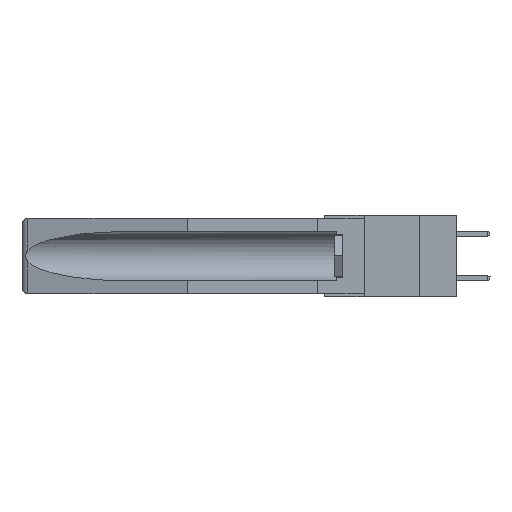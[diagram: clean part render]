
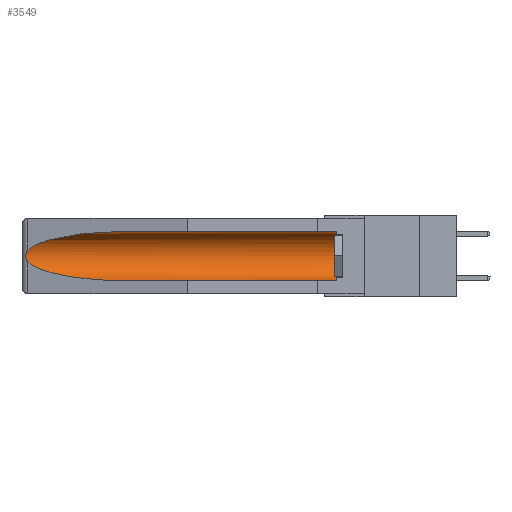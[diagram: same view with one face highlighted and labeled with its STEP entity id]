
A CAD part, left-side view. The second image highlights one B-rep face of the part: STEP entity #3549.
In plain terms, the highlighted cylindrical face has radius 2.857 mm (diameter 5.715 mm), a partial arc.
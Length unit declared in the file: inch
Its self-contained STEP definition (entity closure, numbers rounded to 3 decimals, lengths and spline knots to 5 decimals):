
#280 = CARTESIAN_POINT ( 'NONE',  ( 0.26537, 1.52718, -0.19328 ) ) ;
#306 = DIRECTION ( 'NONE',  ( 0., 1., 0. ) ) ;
#454 = VERTEX_POINT ( 'NONE', #927 ) ;
#563 = CARTESIAN_POINT ( 'NONE',  ( 0.26537, 1.52718, -0.14972 ) ) ;
#865 = DIRECTION ( 'NONE',  ( 0., 1., 0. ) ) ;
#877 = EDGE_LOOP ( 'NONE', ( #3183, #9556, #5149, #1847, #10025, #9889 ) ) ;
#927 = CARTESIAN_POINT ( 'NONE',  ( 0.155, 1.07973, -0.059 ) ) ;
#1046 = CARTESIAN_POINT ( 'NONE',  ( 0.2675, 1.53308, -0.16763 ) ) ;
#1102 = CARTESIAN_POINT ( 'NONE',  ( 0.155, -0.30754, -0.1715 ) ) ;
#1105 = VERTEX_POINT ( 'NONE', #1266 ) ;
#1266 = CARTESIAN_POINT ( 'NONE',  ( 0.155, 0.126, -0.284 ) ) ;
#1847 = ORIENTED_EDGE ( 'NONE', *, *, #3578, .F. ) ;
#2522 = CARTESIAN_POINT ( 'NONE',  ( 0.26597, 1.5296, -0.19026 ) ) ;
#3038 = CARTESIAN_POINT ( 'NONE',  ( 0.155, 0.126, -0.059 ) ) ;
#3183 = ORIENTED_EDGE ( 'NONE', *, *, #11497, .T. ) ;
#3514 = VECTOR ( 'NONE', #306, 39.37008 ) ;
#3549 = ADVANCED_FACE ( 'NONE', ( #17587 ), #16458, .F. ) ;
#3558 = EDGE_CURVE ( 'NONE', #17752, #16629, #10511, .T. ) ;
#3578 = EDGE_CURVE ( 'NONE', #1105, #8417, #11585, .T. ) ;
#3604 = CARTESIAN_POINT ( 'NONE',  ( 0.21114, 1.30732, -0.059 ) ) ;
#3857 = CARTESIAN_POINT ( 'NONE',  ( 0.2675, 1.53308, -0.17534 ) ) ;
#5149 = ORIENTED_EDGE ( 'NONE', *, *, #5478, .T. ) ;
#5207 = CARTESIAN_POINT ( 'NONE',  ( 0.26537, 1.52718, -0.14972 ) ) ;
#5478 = EDGE_CURVE ( 'NONE', #16629, #8417, #10253, .T. ) ;
#5971 = EDGE_CURVE ( 'NONE', #1105, #10099, #11409, .T. ) ;
#6339 = CARTESIAN_POINT ( 'NONE',  ( 0.155, 1.07973, -0.284 ) ) ;
#6468 =( BOUNDED_CURVE ( )  B_SPLINE_CURVE ( 3, ( #11010, #3604, #8084, #563 ),
 .UNSPECIFIED., .F., .F. ) 
 B_SPLINE_CURVE_WITH_KNOTS ( ( 4, 4 ),
 ( 4.71239, 6.08839 ),
 .UNSPECIFIED. ) 
 CURVE ( )  GEOMETRIC_REPRESENTATION_ITEM ( )  RATIONAL_B_SPLINE_CURVE ( ( 1., 0.848, 0.848, 1. ) ) 
 REPRESENTATION_ITEM ( '' )  );
#6842 = CARTESIAN_POINT ( 'NONE',  ( 0.2673, 1.5327, -0.16383 ) ) ;
#7678 = EDGE_CURVE ( 'NONE', #10099, #454, #9026, .T. ) ;
#8084 = CARTESIAN_POINT ( 'NONE',  ( 0.25451, 1.48313, -0.09465 ) ) ;
#8417 = VERTEX_POINT ( 'NONE', #14729 ) ;
#9026 = LINE ( 'NONE', #13500, #3514 ) ;
#9556 = ORIENTED_EDGE ( 'NONE', *, *, #3558, .T. ) ;
#9772 = DIRECTION ( 'NONE',  ( 0., 1., 0. ) ) ;
#9828 = CARTESIAN_POINT ( 'NONE',  ( 0.26597, 1.52961, -0.15275 ) ) ;
#9889 = ORIENTED_EDGE ( 'NONE', *, *, #7678, .T. ) ;
#10025 = ORIENTED_EDGE ( 'NONE', *, *, #5971, .T. ) ;
#10099 = VERTEX_POINT ( 'NONE', #3038 ) ;
#10253 =( BOUNDED_CURVE ( )  B_SPLINE_CURVE ( 3, ( #10804, #16494, #13542, #6339 ),
 .UNSPECIFIED., .F., .F. ) 
 B_SPLINE_CURVE_WITH_KNOTS ( ( 4, 4 ),
 ( 0.1948, 1.5708 ),
 .UNSPECIFIED. ) 
 CURVE ( )  GEOMETRIC_REPRESENTATION_ITEM ( )  RATIONAL_B_SPLINE_CURVE ( ( 1., 0.848, 0.848, 1. ) ) 
 REPRESENTATION_ITEM ( '' )  );
#10511 = B_SPLINE_CURVE_WITH_KNOTS ( 'NONE', 3,
 ( #5207, #9828, #14248, #6842, #1046, #3857, #15685, #15575, #2522, #14193 ),
 .UNSPECIFIED., .F., .F.,
 ( 4, 2, 2, 2, 4 ),
 ( 0., 0.00029, 0.00058, 0.00087, 0.00117 ),
 .UNSPECIFIED. ) ;
#10804 = CARTESIAN_POINT ( 'NONE',  ( 0.26537, 1.52718, -0.19328 ) ) ;
#10883 = DIRECTION ( 'NONE',  ( 0., -1., 0. ) ) ;
#11010 = CARTESIAN_POINT ( 'NONE',  ( 0.155, 1.07973, -0.059 ) ) ;
#11409 = CIRCLE ( 'NONE', #11492, 0.1125 ) ;
#11492 = AXIS2_PLACEMENT_3D ( 'NONE', #16817, #10883, #14111 ) ;
#11497 = EDGE_CURVE ( 'NONE', #454, #17752, #6468, .T. ) ;
#11585 = LINE ( 'NONE', #12826, #16685 ) ;
#12789 = CARTESIAN_POINT ( 'NONE',  ( 0.26537, 1.52718, -0.14972 ) ) ;
#12826 = CARTESIAN_POINT ( 'NONE',  ( 0.155, -0.30754, -0.284 ) ) ;
#13500 = CARTESIAN_POINT ( 'NONE',  ( 0.155, -0.30754, -0.059 ) ) ;
#13542 = CARTESIAN_POINT ( 'NONE',  ( 0.21114, 1.30732, -0.284 ) ) ;
#14111 = DIRECTION ( 'NONE',  ( 0., 0., 1. ) ) ;
#14126 = DIRECTION ( 'NONE',  ( 0., 0., 1. ) ) ;
#14193 = CARTESIAN_POINT ( 'NONE',  ( 0.26537, 1.52718, -0.19328 ) ) ;
#14205 = AXIS2_PLACEMENT_3D ( 'NONE', #1102, #865, #14126 ) ;
#14248 = CARTESIAN_POINT ( 'NONE',  ( 0.26654, 1.53092, -0.15636 ) ) ;
#14729 = CARTESIAN_POINT ( 'NONE',  ( 0.155, 1.07973, -0.284 ) ) ;
#15575 = CARTESIAN_POINT ( 'NONE',  ( 0.26655, 1.53094, -0.18657 ) ) ;
#15685 = CARTESIAN_POINT ( 'NONE',  ( 0.2673, 1.53269, -0.17917 ) ) ;
#16458 = CYLINDRICAL_SURFACE ( 'NONE', #14205, 0.1125 ) ;
#16494 = CARTESIAN_POINT ( 'NONE',  ( 0.25451, 1.48313, -0.24835 ) ) ;
#16629 = VERTEX_POINT ( 'NONE', #280 ) ;
#16685 = VECTOR ( 'NONE', #9772, 39.37008 ) ;
#16817 = CARTESIAN_POINT ( 'NONE',  ( 0.155, 0.126, -0.1715 ) ) ;
#17587 = FACE_OUTER_BOUND ( 'NONE', #877, .T. ) ;
#17752 = VERTEX_POINT ( 'NONE', #12789 ) ;
